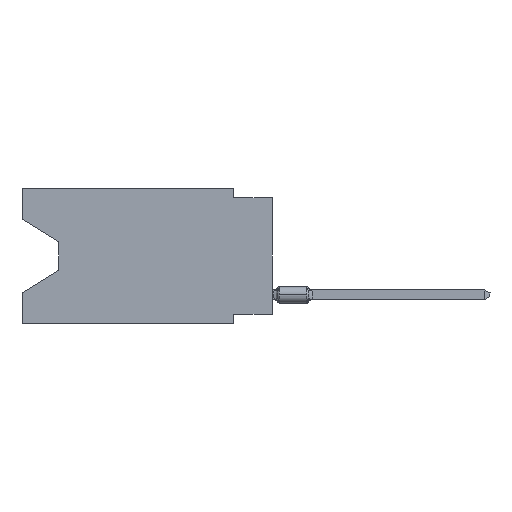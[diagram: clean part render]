
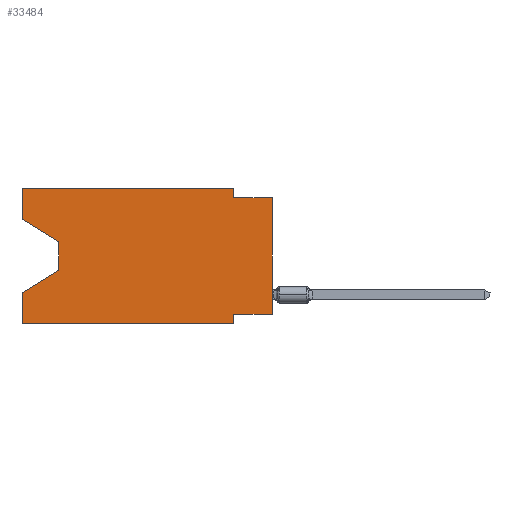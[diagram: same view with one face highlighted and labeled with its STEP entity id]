
A CAD part, left-side view. The second image highlights one B-rep face of the part: STEP entity #33484.
In plain terms, the highlighted planar face has unit normal (-1, 0, 0).
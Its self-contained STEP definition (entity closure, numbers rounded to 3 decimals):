
#407 = LINE ( 'NONE', #21838, #25219 ) ;
#461 = DIRECTION ( 'NONE',  ( 0., -0.855, -0.519 ) ) ;
#2851 = AXIS2_PLACEMENT_3D ( 'NONE', #36643, #47841, #28833 ) ;
#3227 = CARTESIAN_POINT ( 'NONE',  ( 0., 2.54, -8.89 ) ) ;
#4158 = CARTESIAN_POINT ( 'NONE',  ( 0., 16.383, 0. ) ) ;
#4607 = DIRECTION ( 'NONE',  ( 0., 0.855, -0.519 ) ) ;
#4803 = LINE ( 'NONE', #27925, #14309 ) ;
#5696 = CARTESIAN_POINT ( 'NONE',  ( 0., 2.54, -8.255 ) ) ;
#5729 = EDGE_CURVE ( 'NONE', #45798, #37065, #30411, .T. ) ;
#6595 = EDGE_CURVE ( 'NONE', #24891, #37218, #38832, .T. ) ;
#6823 = EDGE_CURVE ( 'NONE', #29895, #37250, #26765, .T. ) ;
#7260 = CARTESIAN_POINT ( 'NONE',  ( 0., 16.383, -2.038 ) ) ;
#7338 = VERTEX_POINT ( 'NONE', #34741 ) ;
#8235 = DIRECTION ( 'NONE',  ( 0., 0., -1. ) ) ;
#8272 = VECTOR ( 'NONE', #16865, 1000. ) ;
#8525 = LINE ( 'NONE', #4158, #25035 ) ;
#8680 = DIRECTION ( 'NONE',  ( 0., 0., 1. ) ) ;
#8820 = EDGE_CURVE ( 'NONE', #28780, #13979, #35286, .T. ) ;
#8846 = VECTOR ( 'NONE', #23908, 1000. ) ;
#9044 = EDGE_CURVE ( 'NONE', #12192, #13979, #407, .T. ) ;
#9408 = VECTOR ( 'NONE', #20800, 1000. ) ;
#9550 = ORIENTED_EDGE ( 'NONE', *, *, #5729, .F. ) ;
#9672 = EDGE_CURVE ( 'NONE', #37218, #7338, #28204, .T. ) ;
#9916 = CARTESIAN_POINT ( 'NONE',  ( 0., 0., -0.635 ) ) ;
#10975 = EDGE_CURVE ( 'NONE', #30374, #7338, #4803, .T. ) ;
#11349 = DIRECTION ( 'NONE',  ( 0., 0., 1. ) ) ;
#12192 = VERTEX_POINT ( 'NONE', #24915 ) ;
#13391 = CARTESIAN_POINT ( 'NONE',  ( 0., 2.54, -0.635 ) ) ;
#13567 = DIRECTION ( 'NONE',  ( 0., -1., 0. ) ) ;
#13979 = VERTEX_POINT ( 'NONE', #36627 ) ;
#14309 = VECTOR ( 'NONE', #8680, 1000. ) ;
#14563 = CARTESIAN_POINT ( 'NONE',  ( 0., 2.54, 0. ) ) ;
#15192 = CARTESIAN_POINT ( 'NONE',  ( 0., 16.383, 0. ) ) ;
#15536 = DIRECTION ( 'NONE',  ( 0., -1., 0. ) ) ;
#15775 = VECTOR ( 'NONE', #13567, 1000. ) ;
#16330 = CARTESIAN_POINT ( 'NONE',  ( 0., 13.97, -3.505 ) ) ;
#16632 = VERTEX_POINT ( 'NONE', #15192 ) ;
#16744 = CARTESIAN_POINT ( 'NONE',  ( 0., 13.97, -5.385 ) ) ;
#16865 = DIRECTION ( 'NONE',  ( 0., 0., -1. ) ) ;
#17860 = FACE_OUTER_BOUND ( 'NONE', #25438, .T. ) ;
#17888 = ORIENTED_EDGE ( 'NONE', *, *, #41765, .F. ) ;
#19116 = LINE ( 'NONE', #41783, #41538 ) ;
#19437 = CARTESIAN_POINT ( 'NONE',  ( 0., 2.54, -8.89 ) ) ;
#19921 = CARTESIAN_POINT ( 'NONE',  ( 0., 16.383, -2.038 ) ) ;
#20038 = ORIENTED_EDGE ( 'NONE', *, *, #38373, .F. ) ;
#20800 = DIRECTION ( 'NONE',  ( 0., 0., 1. ) ) ;
#21118 = EDGE_CURVE ( 'NONE', #12192, #37065, #41639, .T. ) ;
#21838 = CARTESIAN_POINT ( 'NONE',  ( 0., 16.383, 0. ) ) ;
#21982 = PLANE ( 'NONE',  #2851 ) ;
#22318 = ORIENTED_EDGE ( 'NONE', *, *, #6595, .F. ) ;
#23025 = ORIENTED_EDGE ( 'NONE', *, *, #21118, .T. ) ;
#23377 = DIRECTION ( 'NONE',  ( 0., -1., 0. ) ) ;
#23433 = CARTESIAN_POINT ( 'NONE',  ( 0., 0., -8.255 ) ) ;
#23835 = EDGE_CURVE ( 'NONE', #29895, #16632, #24455, .T. ) ;
#23908 = DIRECTION ( 'NONE',  ( 0., 1., 0. ) ) ;
#24455 = LINE ( 'NONE', #39356, #9408 ) ;
#24891 = VERTEX_POINT ( 'NONE', #14563 ) ;
#24915 = CARTESIAN_POINT ( 'NONE',  ( 0., 16.383, -8.89 ) ) ;
#25035 = VECTOR ( 'NONE', #23377, 1000. ) ;
#25219 = VECTOR ( 'NONE', #11349, 1000. ) ;
#25438 = EDGE_LOOP ( 'NONE', ( #37982, #30616, #47643, #30767, #23025, #9550, #20038, #46359, #26646, #22318, #17888, #37857 ) ) ;
#26646 = ORIENTED_EDGE ( 'NONE', *, *, #9672, .F. ) ;
#26765 = LINE ( 'NONE', #19921, #47954 ) ;
#27925 = CARTESIAN_POINT ( 'NONE',  ( 0., 0., 0. ) ) ;
#28204 = LINE ( 'NONE', #9916, #15775 ) ;
#28386 = VECTOR ( 'NONE', #8235, 1000. ) ;
#28780 = VERTEX_POINT ( 'NONE', #30154 ) ;
#28833 = DIRECTION ( 'NONE',  ( 0., 0., -1. ) ) ;
#29895 = VERTEX_POINT ( 'NONE', #7260 ) ;
#30154 = CARTESIAN_POINT ( 'NONE',  ( 0., 13.97, -5.385 ) ) ;
#30374 = VERTEX_POINT ( 'NONE', #38154 ) ;
#30411 = LINE ( 'NONE', #19437, #28386 ) ;
#30616 = ORIENTED_EDGE ( 'NONE', *, *, #45604, .T. ) ;
#30767 = ORIENTED_EDGE ( 'NONE', *, *, #9044, .F. ) ;
#31023 = CARTESIAN_POINT ( 'NONE',  ( 0., 2.54, 0. ) ) ;
#33484 = ADVANCED_FACE ( 'NONE', ( #17860 ), #21982, .F. ) ;
#34741 = CARTESIAN_POINT ( 'NONE',  ( 0., 0., -0.635 ) ) ;
#35286 = LINE ( 'NONE', #16744, #46539 ) ;
#36627 = CARTESIAN_POINT ( 'NONE',  ( 0., 16.383, -6.852 ) ) ;
#36643 = CARTESIAN_POINT ( 'NONE',  ( 0., 16.383, 0. ) ) ;
#37065 = VERTEX_POINT ( 'NONE', #3227 ) ;
#37218 = VERTEX_POINT ( 'NONE', #13391 ) ;
#37250 = VERTEX_POINT ( 'NONE', #16330 ) ;
#37857 = ORIENTED_EDGE ( 'NONE', *, *, #23835, .F. ) ;
#37982 = ORIENTED_EDGE ( 'NONE', *, *, #6823, .T. ) ;
#38154 = CARTESIAN_POINT ( 'NONE',  ( 0., 0., -8.255 ) ) ;
#38373 = EDGE_CURVE ( 'NONE', #30374, #45798, #46588, .T. ) ;
#38832 = LINE ( 'NONE', #31023, #8272 ) ;
#39356 = CARTESIAN_POINT ( 'NONE',  ( 0., 16.383, 0. ) ) ;
#41538 = VECTOR ( 'NONE', #45912, 1000. ) ;
#41639 = LINE ( 'NONE', #45768, #45150 ) ;
#41765 = EDGE_CURVE ( 'NONE', #16632, #24891, #8525, .T. ) ;
#41783 = CARTESIAN_POINT ( 'NONE',  ( 0., 13.97, -3.505 ) ) ;
#45150 = VECTOR ( 'NONE', #15536, 1000. ) ;
#45604 = EDGE_CURVE ( 'NONE', #37250, #28780, #19116, .T. ) ;
#45768 = CARTESIAN_POINT ( 'NONE',  ( 0., 16.383, -8.89 ) ) ;
#45798 = VERTEX_POINT ( 'NONE', #5696 ) ;
#45912 = DIRECTION ( 'NONE',  ( 0., 0., -1. ) ) ;
#46359 = ORIENTED_EDGE ( 'NONE', *, *, #10975, .T. ) ;
#46539 = VECTOR ( 'NONE', #4607, 1000. ) ;
#46588 = LINE ( 'NONE', #23433, #8846 ) ;
#47643 = ORIENTED_EDGE ( 'NONE', *, *, #8820, .T. ) ;
#47841 = DIRECTION ( 'NONE',  ( 1., 0., 0. ) ) ;
#47954 = VECTOR ( 'NONE', #461, 1000. ) ;
